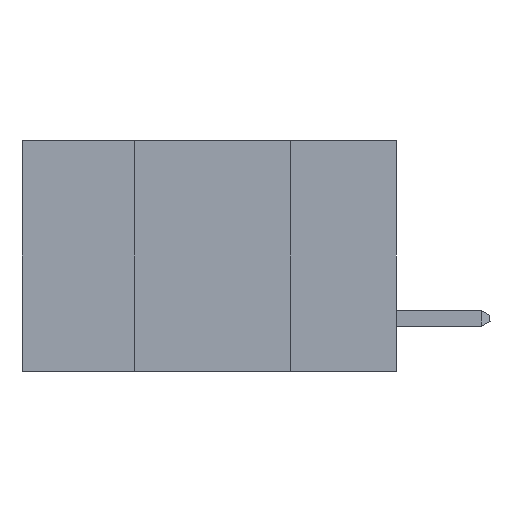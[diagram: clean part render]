
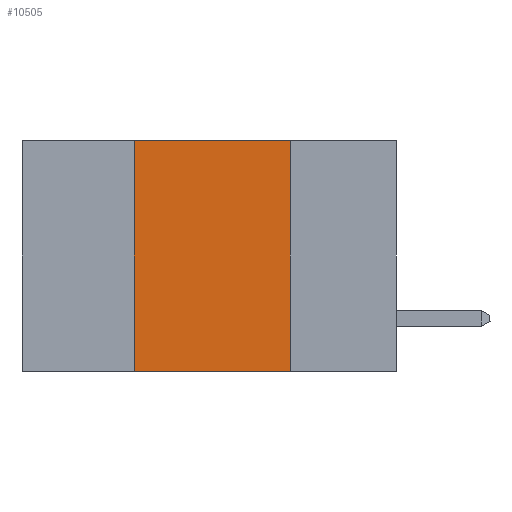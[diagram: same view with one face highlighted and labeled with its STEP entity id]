
A CAD part, left-side view. The second image highlights one B-rep face of the part: STEP entity #10505.
In plain terms, the highlighted planar face has unit normal (-1, 0, 0).
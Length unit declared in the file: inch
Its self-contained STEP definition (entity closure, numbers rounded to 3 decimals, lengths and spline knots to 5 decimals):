
#2377 = VECTOR ( 'NONE', #10656, 39.37008 ) ;
#3746 = VECTOR ( 'NONE', #14994, 39.37008 ) ;
#4053 = CARTESIAN_POINT ( 'NONE',  ( 0., 0.42, 0. ) ) ;
#5139 = LINE ( 'NONE', #28312, #3746 ) ;
#5632 = VECTOR ( 'NONE', #22346, 39.37008 ) ;
#6843 = CARTESIAN_POINT ( 'NONE',  ( 0., 0.17, 0. ) ) ;
#8713 = CARTESIAN_POINT ( 'NONE',  ( 0., 0.6, 0. ) ) ;
#9728 = EDGE_LOOP ( 'NONE', ( #20695, #17542, #12309, #11739 ) ) ;
#9744 = VERTEX_POINT ( 'NONE', #17966 ) ;
#10293 = PLANE ( 'NONE',  #24185 ) ;
#10302 = FACE_OUTER_BOUND ( 'NONE', #9728, .T. ) ;
#10505 = ADVANCED_FACE ( 'NONE', ( #10302 ), #10293, .F. ) ;
#10656 = DIRECTION ( 'NONE',  ( 0., -1., 0. ) ) ;
#11739 = ORIENTED_EDGE ( 'NONE', *, *, #19076, .T. ) ;
#12309 = ORIENTED_EDGE ( 'NONE', *, *, #27825, .F. ) ;
#12346 = DIRECTION ( 'NONE',  ( 1., 0., 0. ) ) ;
#12537 = VECTOR ( 'NONE', #25449, 39.37008 ) ;
#12556 = DIRECTION ( 'NONE',  ( 0., 0., -1. ) ) ;
#14477 = CARTESIAN_POINT ( 'NONE',  ( 0., 0.17, -0.37 ) ) ;
#14635 = CARTESIAN_POINT ( 'NONE',  ( 0., 0.42, 0. ) ) ;
#14994 = DIRECTION ( 'NONE',  ( 0., -1., 0. ) ) ;
#16355 = LINE ( 'NONE', #14635, #12537 ) ;
#16445 = VERTEX_POINT ( 'NONE', #14477 ) ;
#16842 = CARTESIAN_POINT ( 'NONE',  ( 0., 0.6, 0. ) ) ;
#17094 = EDGE_CURVE ( 'NONE', #26156, #9744, #26756, .T. ) ;
#17542 = ORIENTED_EDGE ( 'NONE', *, *, #17094, .F. ) ;
#17966 = CARTESIAN_POINT ( 'NONE',  ( 0., 0.17, 0. ) ) ;
#19076 = EDGE_CURVE ( 'NONE', #25377, #16445, #5139, .T. ) ;
#20255 = LINE ( 'NONE', #6843, #5632 ) ;
#20695 = ORIENTED_EDGE ( 'NONE', *, *, #27191, .F. ) ;
#22346 = DIRECTION ( 'NONE',  ( 0., 0., -1. ) ) ;
#24185 = AXIS2_PLACEMENT_3D ( 'NONE', #16842, #12346, #12556 ) ;
#25377 = VERTEX_POINT ( 'NONE', #28853 ) ;
#25449 = DIRECTION ( 'NONE',  ( 0., 0., 1. ) ) ;
#26156 = VERTEX_POINT ( 'NONE', #4053 ) ;
#26756 = LINE ( 'NONE', #8713, #2377 ) ;
#27191 = EDGE_CURVE ( 'NONE', #9744, #16445, #20255, .T. ) ;
#27825 = EDGE_CURVE ( 'NONE', #25377, #26156, #16355, .T. ) ;
#28312 = CARTESIAN_POINT ( 'NONE',  ( 0., 0.6, -0.37 ) ) ;
#28853 = CARTESIAN_POINT ( 'NONE',  ( 0., 0.42, -0.37 ) ) ;
